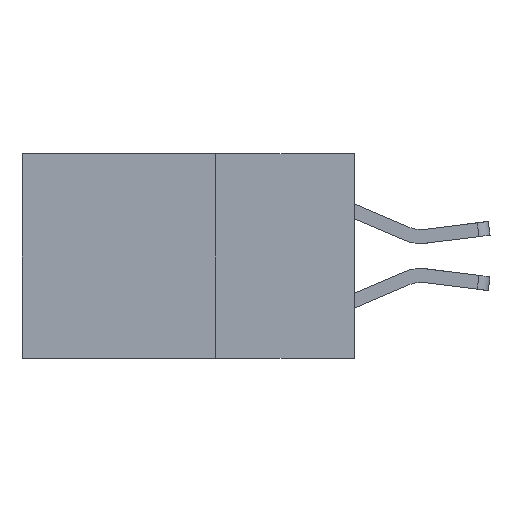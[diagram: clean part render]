
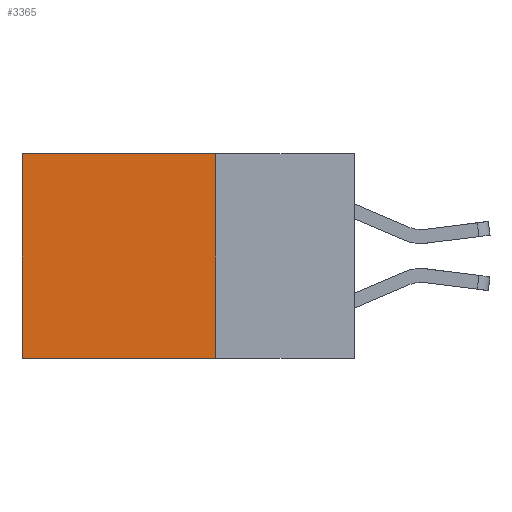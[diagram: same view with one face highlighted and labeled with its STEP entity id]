
A CAD part, left-side view. The second image highlights one B-rep face of the part: STEP entity #3365.
In plain terms, the highlighted planar face has unit normal (-1, 0, 0).
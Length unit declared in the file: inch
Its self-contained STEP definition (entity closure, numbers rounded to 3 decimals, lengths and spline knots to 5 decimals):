
#193 = DIRECTION ( 'NONE',  ( 0., 0., -1. ) ) ;
#404 = VECTOR ( 'NONE', #2847, 39.37008 ) ;
#741 = CARTESIAN_POINT ( 'NONE',  ( 0.2615, 0.25, -0.37 ) ) ;
#927 = DIRECTION ( 'NONE',  ( 0., 1., 0. ) ) ;
#1113 = DIRECTION ( 'NONE',  ( 0., 1., 0. ) ) ;
#1151 = CARTESIAN_POINT ( 'NONE',  ( 0.2615, 0.25, -0.37 ) ) ;
#1219 = EDGE_CURVE ( 'NONE', #5919, #3930, #8460, .T. ) ;
#1288 = VECTOR ( 'NONE', #927, 39.37008 ) ;
#1466 = VECTOR ( 'NONE', #1113, 39.37008 ) ;
#1987 = FACE_OUTER_BOUND ( 'NONE', #4119, .T. ) ;
#2440 = CARTESIAN_POINT ( 'NONE',  ( 0.2615, 0.25, -0.37 ) ) ;
#2698 = DIRECTION ( 'NONE',  ( 0., 0., -1. ) ) ;
#2847 = DIRECTION ( 'NONE',  ( 0., 0., -1. ) ) ;
#3261 = CARTESIAN_POINT ( 'NONE',  ( 0.2615, 0.6, 0. ) ) ;
#3343 = ORIENTED_EDGE ( 'NONE', *, *, #8149, .F. ) ;
#3365 = ADVANCED_FACE ( 'NONE', ( #1987 ), #3367, .F. ) ;
#3367 = PLANE ( 'NONE',  #4597 ) ;
#3608 = LINE ( 'NONE', #4863, #404 ) ;
#3865 = DIRECTION ( 'NONE',  ( 1., 0., 0. ) ) ;
#3914 = CARTESIAN_POINT ( 'NONE',  ( 0.2615, 0.25, 0. ) ) ;
#3930 = VERTEX_POINT ( 'NONE', #6986 ) ;
#4119 = EDGE_LOOP ( 'NONE', ( #8130, #7168, #3343, #4688 ) ) ;
#4332 = LINE ( 'NONE', #7059, #1288 ) ;
#4597 = AXIS2_PLACEMENT_3D ( 'NONE', #1151, #3865, #2698 ) ;
#4688 = ORIENTED_EDGE ( 'NONE', *, *, #5058, .T. ) ;
#4737 = VECTOR ( 'NONE', #193, 39.37008 ) ;
#4863 = CARTESIAN_POINT ( 'NONE',  ( 0.2615, 0.6, -0.37 ) ) ;
#4994 = EDGE_CURVE ( 'NONE', #8703, #3930, #3608, .T. ) ;
#5058 = EDGE_CURVE ( 'NONE', #5268, #8703, #4332, .T. ) ;
#5268 = VERTEX_POINT ( 'NONE', #3914 ) ;
#5919 = VERTEX_POINT ( 'NONE', #7928 ) ;
#6259 = LINE ( 'NONE', #741, #4737 ) ;
#6986 = CARTESIAN_POINT ( 'NONE',  ( 0.2615, 0.6, -0.37 ) ) ;
#7059 = CARTESIAN_POINT ( 'NONE',  ( 0.2615, 0.25, 0. ) ) ;
#7168 = ORIENTED_EDGE ( 'NONE', *, *, #1219, .F. ) ;
#7928 = CARTESIAN_POINT ( 'NONE',  ( 0.2615, 0.25, -0.37 ) ) ;
#8130 = ORIENTED_EDGE ( 'NONE', *, *, #4994, .T. ) ;
#8149 = EDGE_CURVE ( 'NONE', #5268, #5919, #6259, .T. ) ;
#8460 = LINE ( 'NONE', #2440, #1466 ) ;
#8703 = VERTEX_POINT ( 'NONE', #3261 ) ;
